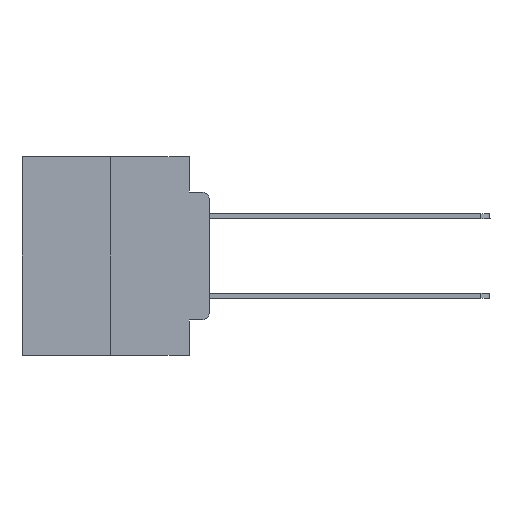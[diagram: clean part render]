
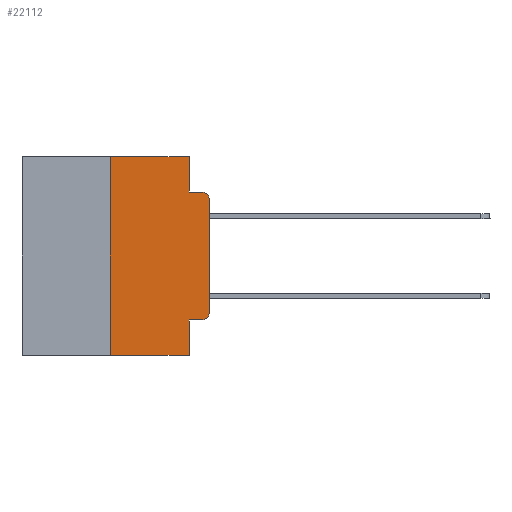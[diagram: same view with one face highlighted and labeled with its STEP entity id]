
A CAD part, left-side view. The second image highlights one B-rep face of the part: STEP entity #22112.
In plain terms, the highlighted planar face has unit normal (-1, 0, 0).
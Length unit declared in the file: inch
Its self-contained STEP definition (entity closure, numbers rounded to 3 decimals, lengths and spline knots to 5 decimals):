
#185 = VERTEX_POINT ( 'NONE', #24347 ) ;
#317 = CARTESIAN_POINT ( 'NONE',  ( 0., 0.051, 0. ) ) ;
#496 = VECTOR ( 'NONE', #23219, 39.37008 ) ;
#1404 = CARTESIAN_POINT ( 'NONE',  ( 0., 0., -0.3915 ) ) ;
#4940 = EDGE_CURVE ( 'NONE', #12044, #19688, #10345, .T. ) ;
#5609 = ORIENTED_EDGE ( 'NONE', *, *, #8511, .F. ) ;
#5838 = CARTESIAN_POINT ( 'NONE',  ( 0., 0.473, 0. ) ) ;
#5984 = EDGE_LOOP ( 'NONE', ( #11906, #12958, #9219, #18681, #5609, #18192, #10061, #21671, #15311, #7827 ) ) ;
#6116 = DIRECTION ( 'NONE',  ( 0., -1., 0. ) ) ;
#6565 = DIRECTION ( 'NONE',  ( 0., 0., -1. ) ) ;
#6807 = DIRECTION ( 'NONE',  ( -1., 0., 0. ) ) ;
#7287 = LINE ( 'NONE', #19264, #496 ) ;
#7374 = DIRECTION ( 'NONE',  ( 0., 0., 1. ) ) ;
#7403 = VERTEX_POINT ( 'NONE', #15047 ) ;
#7586 = CARTESIAN_POINT ( 'NONE',  ( 0., 0.02, -0.1085 ) ) ;
#7600 = CARTESIAN_POINT ( 'NONE',  ( 0., 0.051, -0.0885 ) ) ;
#7827 = ORIENTED_EDGE ( 'NONE', *, *, #4940, .T. ) ;
#7946 = EDGE_CURVE ( 'NONE', #25694, #7403, #23334, .T. ) ;
#8054 = VECTOR ( 'NONE', #14392, 39.37008 ) ;
#8061 = CARTESIAN_POINT ( 'NONE',  ( 0., 0.02, -0.0885 ) ) ;
#8511 = EDGE_CURVE ( 'NONE', #22067, #17329, #7287, .T. ) ;
#9219 = ORIENTED_EDGE ( 'NONE', *, *, #20883, .F. ) ;
#9427 = CARTESIAN_POINT ( 'NONE',  ( 0., 0., 0. ) ) ;
#9634 = LINE ( 'NONE', #7600, #20141 ) ;
#9698 = DIRECTION ( 'NONE',  ( 0., 0., -1. ) ) ;
#10061 = ORIENTED_EDGE ( 'NONE', *, *, #7946, .T. ) ;
#10125 = EDGE_CURVE ( 'NONE', #25694, #22067, #15299, .T. ) ;
#10345 = CIRCLE ( 'NONE', #16897, 0.02 ) ;
#10804 = CARTESIAN_POINT ( 'NONE',  ( 0., 0.051, 0. ) ) ;
#11454 = CARTESIAN_POINT ( 'NONE',  ( 0., 0.051, -0.4115 ) ) ;
#11512 = FACE_OUTER_BOUND ( 'NONE', #5984, .T. ) ;
#11906 = ORIENTED_EDGE ( 'NONE', *, *, #12219, .T. ) ;
#12044 = VERTEX_POINT ( 'NONE', #24717 ) ;
#12050 = CARTESIAN_POINT ( 'NONE',  ( 0., 0.25, 0. ) ) ;
#12219 = EDGE_CURVE ( 'NONE', #19688, #16953, #12657, .T. ) ;
#12311 = VECTOR ( 'NONE', #13131, 39.37008 ) ;
#12560 = CARTESIAN_POINT ( 'NONE',  ( 0., 0.473, -0.5 ) ) ;
#12657 = LINE ( 'NONE', #9427, #17434 ) ;
#12958 = ORIENTED_EDGE ( 'NONE', *, *, #19137, .T. ) ;
#13131 = DIRECTION ( 'NONE',  ( 0., 0., -1. ) ) ;
#13382 = CARTESIAN_POINT ( 'NONE',  ( 0., 0.051, -0.4115 ) ) ;
#14392 = DIRECTION ( 'NONE',  ( 0., 0., -1. ) ) ;
#15047 = CARTESIAN_POINT ( 'NONE',  ( 0., 0.051, -0.5 ) ) ;
#15299 = LINE ( 'NONE', #19612, #17238 ) ;
#15311 = ORIENTED_EDGE ( 'NONE', *, *, #23117, .T. ) ;
#16897 = AXIS2_PLACEMENT_3D ( 'NONE', #17098, #6807, #6565 ) ;
#16953 = VERTEX_POINT ( 'NONE', #23000 ) ;
#17098 = CARTESIAN_POINT ( 'NONE',  ( 0., 0.02, -0.3915 ) ) ;
#17166 = DIRECTION ( 'NONE',  ( 0., -1., 0. ) ) ;
#17238 = VECTOR ( 'NONE', #23927, 39.37008 ) ;
#17329 = VERTEX_POINT ( 'NONE', #317 ) ;
#17391 = CIRCLE ( 'NONE', #24048, 0.02 ) ;
#17434 = VECTOR ( 'NONE', #7374, 39.37008 ) ;
#17867 = VECTOR ( 'NONE', #6116, 39.37008 ) ;
#18192 = ORIENTED_EDGE ( 'NONE', *, *, #10125, .F. ) ;
#18681 = ORIENTED_EDGE ( 'NONE', *, *, #20559, .F. ) ;
#18686 = CARTESIAN_POINT ( 'NONE',  ( 0., 0.051, 0. ) ) ;
#18798 = EDGE_CURVE ( 'NONE', #21945, #7403, #23192, .T. ) ;
#19137 = EDGE_CURVE ( 'NONE', #16953, #20742, #17391, .T. ) ;
#19192 = AXIS2_PLACEMENT_3D ( 'NONE', #5838, #20135, #9698 ) ;
#19264 = CARTESIAN_POINT ( 'NONE',  ( 0., 0.473, 0. ) ) ;
#19612 = CARTESIAN_POINT ( 'NONE',  ( 0., 0.25, 0. ) ) ;
#19688 = VERTEX_POINT ( 'NONE', #1404 ) ;
#19964 = PLANE ( 'NONE',  #19192 ) ;
#20135 = DIRECTION ( 'NONE',  ( 1., 0., 0. ) ) ;
#20141 = VECTOR ( 'NONE', #21889, 39.37008 ) ;
#20559 = EDGE_CURVE ( 'NONE', #17329, #185, #20848, .T. ) ;
#20742 = VERTEX_POINT ( 'NONE', #8061 ) ;
#20848 = LINE ( 'NONE', #18686, #8054 ) ;
#20883 = EDGE_CURVE ( 'NONE', #185, #20742, #9634, .T. ) ;
#21671 = ORIENTED_EDGE ( 'NONE', *, *, #18798, .F. ) ;
#21889 = DIRECTION ( 'NONE',  ( 0., -1., 0. ) ) ;
#21945 = VERTEX_POINT ( 'NONE', #13382 ) ;
#21976 = DIRECTION ( 'NONE',  ( 0., 0., -1. ) ) ;
#22067 = VERTEX_POINT ( 'NONE', #12050 ) ;
#22112 = ADVANCED_FACE ( 'NONE', ( #11512 ), #19964, .F. ) ;
#23000 = CARTESIAN_POINT ( 'NONE',  ( 0., 0., -0.1085 ) ) ;
#23117 = EDGE_CURVE ( 'NONE', #21945, #12044, #26185, .T. ) ;
#23192 = LINE ( 'NONE', #10804, #12311 ) ;
#23219 = DIRECTION ( 'NONE',  ( 0., -1., 0. ) ) ;
#23334 = LINE ( 'NONE', #12560, #17867 ) ;
#23632 = VECTOR ( 'NONE', #17166, 39.37008 ) ;
#23901 = CARTESIAN_POINT ( 'NONE',  ( 0., 0.25, -0.5 ) ) ;
#23927 = DIRECTION ( 'NONE',  ( 0., 0., 1. ) ) ;
#24048 = AXIS2_PLACEMENT_3D ( 'NONE', #7586, #26263, #21976 ) ;
#24347 = CARTESIAN_POINT ( 'NONE',  ( 0., 0.051, -0.0885 ) ) ;
#24717 = CARTESIAN_POINT ( 'NONE',  ( 0., 0.02, -0.4115 ) ) ;
#25694 = VERTEX_POINT ( 'NONE', #23901 ) ;
#26185 = LINE ( 'NONE', #11454, #23632 ) ;
#26263 = DIRECTION ( 'NONE',  ( -1., 0., 0. ) ) ;
